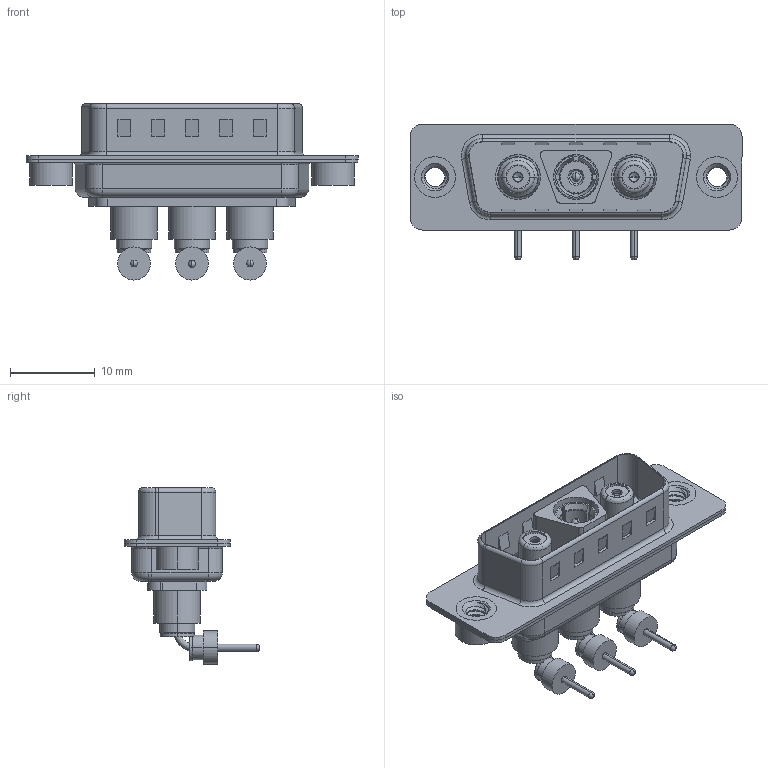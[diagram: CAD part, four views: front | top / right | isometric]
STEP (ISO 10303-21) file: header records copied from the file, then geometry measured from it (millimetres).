
FILE_DESCRIPTION (( 'STEP AP203' ), '1' );
FILE_NAME ('629-3WK3240-5N2.STEP', '2022-05-05T09:42:15', ( '' ), ( '' ), 'SwSTEP 2.0', 'SolidWorks 2020', '' );
FILE_SCHEMA (( 'CONFIG_CONTROL_DESIGN' ));
Length unit declared in the file: millimetre
Products named in the file (17): Insulator Socket 2; Insulator Pin_Straight PC Tail; 629-3WK3240-5N2; Co-Ax Jack Assy_RA; 629Combo Housing_3WK3; 629Combo Shell Front_15 Contacts; Insulator RA Pin; Co-Ax Plug_RA PC Tail; Co-Ax Jack_RA PC Tail; Socket_RA; Insulator Socket; Pin_RA; 629Combo Shell Rear_15 Contacts; Locking Collar; 629Combo Threaded Rivet_2; Co-Ax Plug Assy_RA
Assembly tree (25 placements, depth 3):
  629-3WK3240-5N2
    629Combo Housing_3WK3
    629Combo Shell Rear_15 Contacts
    629Combo Shell Front_15 Contacts
    629Combo Threaded Rivet_2  x2
    Co-Ax Plug Assy_RA
      Co-Ax Plug_RA PC Tail
      Insulator Pin_Straight PC Tail
      Pin_RA
      Locking Collar
      Insulator RA Pin
    Co-Ax Jack Assy_RA
      Co-Ax Jack_RA PC Tail
      Insulator Socket
      Insulator Socket 2
      Locking Collar
      Socket_RA
      Insulator RA Pin
    Co-Ax Jack Assy_RA
      Co-Ax Jack_RA PC Tail
      Insulator Socket
      Insulator Socket 2
      Locking Collar
      Socket_RA
      Insulator RA Pin
Bounding box: 39.2 x 16 x 20.79 mm (x, y, z)
Volume: 2275.6 mm3; surface area: 6625.8 mm2
Topology: 22 solids, 22 shells, 717 faces, 1714 edges, 1080 vertices
Faces by surface type: cylinder 319, plane 256, torus 68, cone 57, bspline 9, sphere 8
Entity records: 19830 total; most frequent: CARTESIAN_POINT 4450, DIRECTION 2992, ORIENTED_EDGE 2650, EDGE_CURVE 1325, AXIS2_PLACEMENT_3D 1165, VERTEX_POINT 840, LINE 662, VECTOR 662
